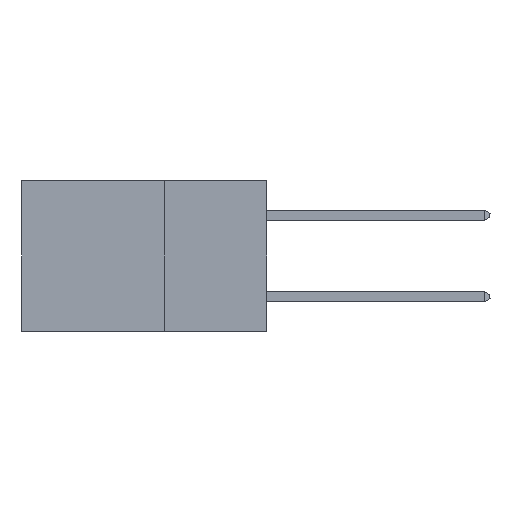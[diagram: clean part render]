
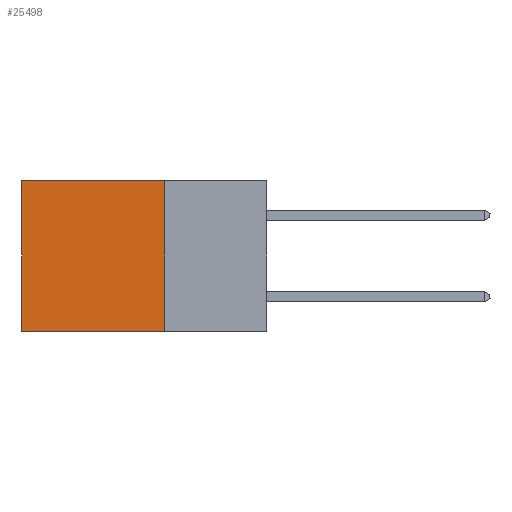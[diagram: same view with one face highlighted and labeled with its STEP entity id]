
A CAD part, left-side view. The second image highlights one B-rep face of the part: STEP entity #25498.
In plain terms, the highlighted planar face has unit normal (-1, 0, 0).
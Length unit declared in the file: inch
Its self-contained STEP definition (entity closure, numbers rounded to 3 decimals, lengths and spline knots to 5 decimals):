
#79 = CARTESIAN_POINT ( 'NONE',  ( 0.2875, 0.25, -0.37 ) ) ;
#1172 = LINE ( 'NONE', #30732, #14545 ) ;
#3420 = CARTESIAN_POINT ( 'NONE',  ( 0.2875, 0.25, 0. ) ) ;
#3907 = VERTEX_POINT ( 'NONE', #79 ) ;
#6901 = VERTEX_POINT ( 'NONE', #17059 ) ;
#7581 = ORIENTED_EDGE ( 'NONE', *, *, #24056, .T. ) ;
#8151 = DIRECTION ( 'NONE',  ( 0., 1., 0. ) ) ;
#10299 = DIRECTION ( 'NONE',  ( 1., 0., 0. ) ) ;
#11465 = VECTOR ( 'NONE', #8151, 39.37008 ) ;
#12120 = CARTESIAN_POINT ( 'NONE',  ( 0.2875, 0.25, 0. ) ) ;
#13559 = VERTEX_POINT ( 'NONE', #26791 ) ;
#14083 = EDGE_LOOP ( 'NONE', ( #7581, #29174, #16543, #32135 ) ) ;
#14545 = VECTOR ( 'NONE', #33222, 39.37008 ) ;
#14873 = CARTESIAN_POINT ( 'NONE',  ( 0.2875, 0.6, 0. ) ) ;
#15251 = PLANE ( 'NONE',  #18115 ) ;
#15866 = EDGE_CURVE ( 'NONE', #3907, #13559, #33431, .T. ) ;
#16543 = ORIENTED_EDGE ( 'NONE', *, *, #32910, .F. ) ;
#17059 = CARTESIAN_POINT ( 'NONE',  ( 0.2875, 0.6, 0. ) ) ;
#18115 = AXIS2_PLACEMENT_3D ( 'NONE', #20381, #10299, #25390 ) ;
#18474 = FACE_OUTER_BOUND ( 'NONE', #14083, .T. ) ;
#20381 = CARTESIAN_POINT ( 'NONE',  ( 0.2875, 0.25, 0. ) ) ;
#20752 = CARTESIAN_POINT ( 'NONE',  ( 0.2875, 0.25, -0.37 ) ) ;
#21083 = VECTOR ( 'NONE', #27830, 39.37008 ) ;
#23304 = VECTOR ( 'NONE', #25507, 39.37008 ) ;
#24056 = EDGE_CURVE ( 'NONE', #6901, #13559, #32422, .T. ) ;
#25390 = DIRECTION ( 'NONE',  ( 0., 0., -1. ) ) ;
#25498 = ADVANCED_FACE ( 'NONE', ( #18474 ), #15251, .F. ) ;
#25507 = DIRECTION ( 'NONE',  ( 0., 1., 0. ) ) ;
#26651 = VERTEX_POINT ( 'NONE', #3420 ) ;
#26791 = CARTESIAN_POINT ( 'NONE',  ( 0.2875, 0.6, -0.37 ) ) ;
#26910 = LINE ( 'NONE', #12120, #11465 ) ;
#27830 = DIRECTION ( 'NONE',  ( 0., 0., -1. ) ) ;
#29174 = ORIENTED_EDGE ( 'NONE', *, *, #15866, .F. ) ;
#30401 = EDGE_CURVE ( 'NONE', #26651, #6901, #26910, .T. ) ;
#30732 = CARTESIAN_POINT ( 'NONE',  ( 0.2875, 0.25, 0. ) ) ;
#32135 = ORIENTED_EDGE ( 'NONE', *, *, #30401, .T. ) ;
#32422 = LINE ( 'NONE', #14873, #21083 ) ;
#32910 = EDGE_CURVE ( 'NONE', #26651, #3907, #1172, .T. ) ;
#33222 = DIRECTION ( 'NONE',  ( 0., 0., -1. ) ) ;
#33431 = LINE ( 'NONE', #20752, #23304 ) ;
